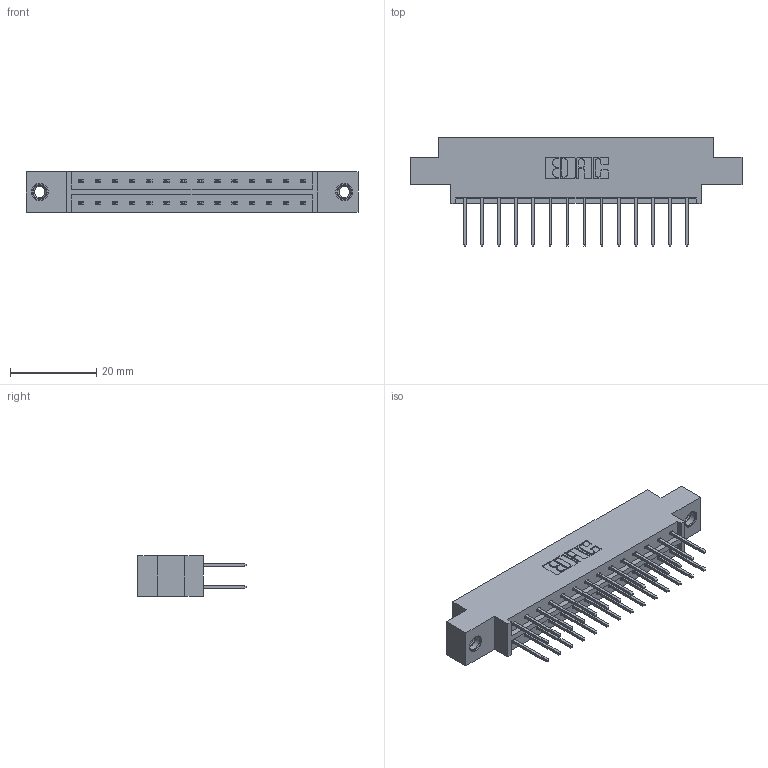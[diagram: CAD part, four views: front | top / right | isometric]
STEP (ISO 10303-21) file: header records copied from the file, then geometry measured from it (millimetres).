
FILE_DESCRIPTION (( 'STEP AP203' ), '1' );
FILE_NAME ('833-028-523-807.STEP', '2020-06-02T08:15:40', ( '' ), ( '' ), 'SwSTEP 2.0', 'SolidWorks 2020', '' );
FILE_SCHEMA (( 'CONFIG_CONTROL_DESIGN' ));
Length unit declared in the file: inch
Products named in the file (4): 833-028-523-807; 345-250-001_345-250-005-103; 833 Part_Offset - .156 Dia - TI; 345-292-001_345-293-123
Assembly tree (31 placements, depth 2):
  833-028-523-807
    833 Part_Offset - .156 Dia - TI
    345-292-001_345-293-123  x28
    345-250-001_345-250-005-103  x2
Bounding box: 77.01 x 25.15 x 9.4 mm (x, y, z)
Volume: 7416.8 mm3; surface area: 8994.2 mm2
Topology: 31 solids, 31 shells, 1634 faces, 4799 edges, 3154 vertices
Faces by surface type: plane 1114, cylinder 504, cone 12, torus 4
Entity records: 13964 total; most frequent: CARTESIAN_POINT 2333, ORIENTED_EDGE 2262, DIRECTION 2073, EDGE_CURVE 1131, VECTOR 983, LINE 983, VERTEX_POINT 748, AXIS2_PLACEMENT_3D 545
